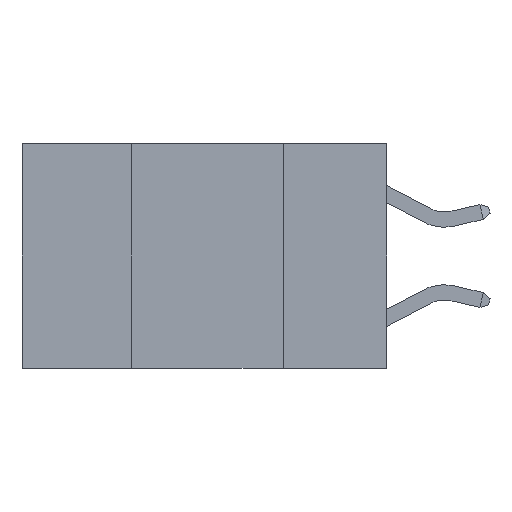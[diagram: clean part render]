
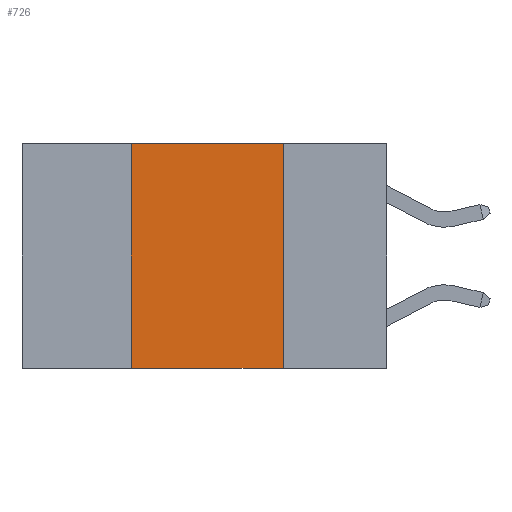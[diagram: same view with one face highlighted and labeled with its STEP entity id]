
A CAD part, left-side view. The second image highlights one B-rep face of the part: STEP entity #726.
In plain terms, the highlighted planar face has unit normal (-1, 0, 0).
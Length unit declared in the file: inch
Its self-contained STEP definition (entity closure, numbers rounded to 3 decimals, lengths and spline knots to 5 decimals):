
#726 = ADVANCED_FACE ( 'NONE', ( #5477 ), #7526, .F. ) ;
#907 = CARTESIAN_POINT ( 'NONE',  ( 0., 0.42, -0.37 ) ) ;
#1070 = ORIENTED_EDGE ( 'NONE', *, *, #1693, .F. ) ;
#1412 = CARTESIAN_POINT ( 'NONE',  ( 0., 0.6, 0. ) ) ;
#1578 = DIRECTION ( 'NONE',  ( 1., 0., 0. ) ) ;
#1643 = VECTOR ( 'NONE', #10877, 39.37008 ) ;
#1693 = EDGE_CURVE ( 'NONE', #2119, #6197, #7073, .T. ) ;
#2066 = VECTOR ( 'NONE', #10198, 39.37008 ) ;
#2119 = VERTEX_POINT ( 'NONE', #907 ) ;
#2317 = EDGE_CURVE ( 'NONE', #10887, #8438, #9298, .T. ) ;
#5453 = ORIENTED_EDGE ( 'NONE', *, *, #11295, .F. ) ;
#5477 = FACE_OUTER_BOUND ( 'NONE', #11810, .T. ) ;
#5550 = DIRECTION ( 'NONE',  ( 0., 0., -1. ) ) ;
#5848 = CARTESIAN_POINT ( 'NONE',  ( 0., 0.42, 0. ) ) ;
#6197 = VERTEX_POINT ( 'NONE', #5848 ) ;
#7073 = LINE ( 'NONE', #7189, #1643 ) ;
#7103 = CARTESIAN_POINT ( 'NONE',  ( 0., 0.17, -0.37 ) ) ;
#7189 = CARTESIAN_POINT ( 'NONE',  ( 0., 0.42, 0. ) ) ;
#7487 = LINE ( 'NONE', #1412, #10726 ) ;
#7526 = PLANE ( 'NONE',  #10213 ) ;
#7803 = LINE ( 'NONE', #12656, #10947 ) ;
#8438 = VERTEX_POINT ( 'NONE', #7103 ) ;
#8677 = ORIENTED_EDGE ( 'NONE', *, *, #12552, .T. ) ;
#8795 = DIRECTION ( 'NONE',  ( 0., -1., 0. ) ) ;
#9104 = CARTESIAN_POINT ( 'NONE',  ( 0., 0.17, 0. ) ) ;
#9249 = DIRECTION ( 'NONE',  ( 0., -1., 0. ) ) ;
#9298 = LINE ( 'NONE', #9104, #2066 ) ;
#10198 = DIRECTION ( 'NONE',  ( 0., 0., -1. ) ) ;
#10213 = AXIS2_PLACEMENT_3D ( 'NONE', #10376, #1578, #5550 ) ;
#10376 = CARTESIAN_POINT ( 'NONE',  ( 0., 0.6, 0. ) ) ;
#10503 = CARTESIAN_POINT ( 'NONE',  ( 0., 0.17, 0. ) ) ;
#10726 = VECTOR ( 'NONE', #9249, 39.37008 ) ;
#10877 = DIRECTION ( 'NONE',  ( 0., 0., 1. ) ) ;
#10887 = VERTEX_POINT ( 'NONE', #10503 ) ;
#10947 = VECTOR ( 'NONE', #8795, 39.37008 ) ;
#11295 = EDGE_CURVE ( 'NONE', #6197, #10887, #7487, .T. ) ;
#11810 = EDGE_LOOP ( 'NONE', ( #12039, #5453, #1070, #8677 ) ) ;
#12039 = ORIENTED_EDGE ( 'NONE', *, *, #2317, .F. ) ;
#12552 = EDGE_CURVE ( 'NONE', #2119, #8438, #7803, .T. ) ;
#12656 = CARTESIAN_POINT ( 'NONE',  ( 0., 0.6, -0.37 ) ) ;
